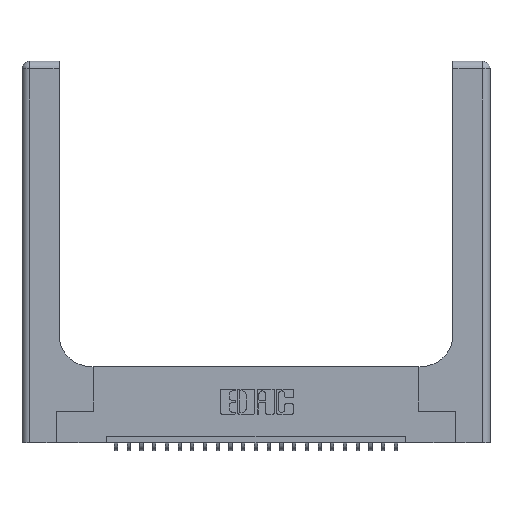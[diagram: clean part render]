
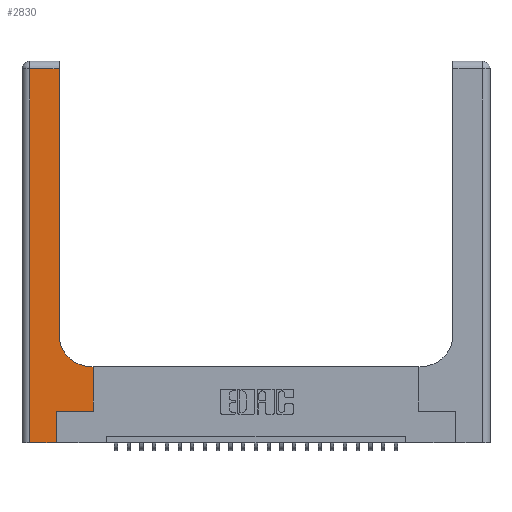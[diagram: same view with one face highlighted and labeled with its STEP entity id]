
A CAD part, top view. The second image highlights one B-rep face of the part: STEP entity #2830.
In plain terms, the highlighted planar face has unit normal (0, 0, 1).
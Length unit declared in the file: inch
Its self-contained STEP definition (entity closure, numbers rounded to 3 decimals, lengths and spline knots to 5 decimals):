
#222 = VERTEX_POINT ( 'NONE', #19089 ) ;
#286 = DIRECTION ( 'NONE',  ( 0., 1., 0. ) ) ;
#414 = CARTESIAN_POINT ( 'NONE',  ( 0.5415, 0.6, 0.37 ) ) ;
#593 = LINE ( 'NONE', #1407, #20966 ) ;
#1171 = CARTESIAN_POINT ( 'NONE',  ( 0.5585, 0.25, 0.37 ) ) ;
#1226 = FACE_OUTER_BOUND ( 'NONE', #12629, .T. ) ;
#1344 = LINE ( 'NONE', #21145, #14712 ) ;
#1407 = CARTESIAN_POINT ( 'NONE',  ( 0.06, 3., 0.37 ) ) ;
#2830 = ADVANCED_FACE ( 'NONE', ( #1226 ), #5696, .F. ) ;
#3647 = DIRECTION ( 'NONE',  ( -1., 0., 0. ) ) ;
#3951 = LINE ( 'NONE', #14547, #21245 ) ;
#5026 = ORIENTED_EDGE ( 'NONE', *, *, #21428, .T. ) ;
#5263 = VERTEX_POINT ( 'NONE', #8131 ) ;
#5564 = CARTESIAN_POINT ( 'NONE',  ( 0.5585, 0.25, 0.37 ) ) ;
#5696 = PLANE ( 'NONE',  #17674 ) ;
#5729 = ORIENTED_EDGE ( 'NONE', *, *, #15155, .T. ) ;
#6501 = VECTOR ( 'NONE', #286, 39.37008 ) ;
#6520 = LINE ( 'NONE', #1171, #6821 ) ;
#6821 = VECTOR ( 'NONE', #14760, 39.37008 ) ;
#7283 = EDGE_CURVE ( 'NONE', #222, #21308, #1344, .T. ) ;
#7438 = ORIENTED_EDGE ( 'NONE', *, *, #7283, .T. ) ;
#7565 = DIRECTION ( 'NONE',  ( 0., 0., -1. ) ) ;
#7624 = EDGE_CURVE ( 'NONE', #19038, #5263, #6520, .T. ) ;
#8131 = CARTESIAN_POINT ( 'NONE',  ( 0.5585, 0.6, 0.37 ) ) ;
#8692 = VERTEX_POINT ( 'NONE', #13277 ) ;
#9406 = CARTESIAN_POINT ( 'NONE',  ( 0., 0., 0.37 ) ) ;
#10143 = DIRECTION ( 'NONE',  ( 0., -1., 0. ) ) ;
#10182 = LINE ( 'NONE', #21748, #13171 ) ;
#10460 = ORIENTED_EDGE ( 'NONE', *, *, #20846, .T. ) ;
#11235 = DIRECTION ( 'NONE',  ( -1., 0., 0. ) ) ;
#12629 = EDGE_LOOP ( 'NONE', ( #7438, #10460, #18470, #15823, #5026, #5729, #13720, #17035, #15009 ) ) ;
#13171 = VECTOR ( 'NONE', #19708, 39.37008 ) ;
#13198 = LINE ( 'NONE', #13828, #19577 ) ;
#13277 = CARTESIAN_POINT ( 'NONE',  ( 0.06, 2.94, 0.37 ) ) ;
#13284 = CARTESIAN_POINT ( 'NONE',  ( 0., 3., 0.37 ) ) ;
#13365 = DIRECTION ( 'NONE',  ( 1., 0., 0. ) ) ;
#13601 = EDGE_CURVE ( 'NONE', #8692, #20129, #593, .T. ) ;
#13603 = CARTESIAN_POINT ( 'NONE',  ( 0.06, 0., 0.37 ) ) ;
#13720 = ORIENTED_EDGE ( 'NONE', *, *, #7624, .T. ) ;
#13828 = CARTESIAN_POINT ( 'NONE',  ( 0., 2.94, 0.37 ) ) ;
#14547 = CARTESIAN_POINT ( 'NONE',  ( 0.2915, 0.6, 0.37 ) ) ;
#14712 = VECTOR ( 'NONE', #22894, 39.37008 ) ;
#14760 = DIRECTION ( 'NONE',  ( 0., 1., 0. ) ) ;
#14888 = CARTESIAN_POINT ( 'NONE',  ( 0.269, 0., 0.37 ) ) ;
#15009 = ORIENTED_EDGE ( 'NONE', *, *, #15524, .T. ) ;
#15155 = EDGE_CURVE ( 'NONE', #17272, #19038, #10182, .T. ) ;
#15264 = VERTEX_POINT ( 'NONE', #414 ) ;
#15524 = EDGE_CURVE ( 'NONE', #15264, #222, #21955, .T. ) ;
#15766 = DIRECTION ( 'NONE',  ( -1., 0., 0. ) ) ;
#15823 = ORIENTED_EDGE ( 'NONE', *, *, #16827, .T. ) ;
#15845 = LINE ( 'NONE', #9406, #20418 ) ;
#16827 = EDGE_CURVE ( 'NONE', #20129, #23615, #15845, .T. ) ;
#17035 = ORIENTED_EDGE ( 'NONE', *, *, #18472, .T. ) ;
#17272 = VERTEX_POINT ( 'NONE', #20364 ) ;
#17674 = AXIS2_PLACEMENT_3D ( 'NONE', #13284, #7565, #3647 ) ;
#18016 = DIRECTION ( 'NONE',  ( 0., 0., -1. ) ) ;
#18470 = ORIENTED_EDGE ( 'NONE', *, *, #13601, .T. ) ;
#18472 = EDGE_CURVE ( 'NONE', #5263, #15264, #3951, .T. ) ;
#19038 = VERTEX_POINT ( 'NONE', #5564 ) ;
#19089 = CARTESIAN_POINT ( 'NONE',  ( 0.2915, 0.85, 0.37 ) ) ;
#19577 = VECTOR ( 'NONE', #15766, 39.37008 ) ;
#19708 = DIRECTION ( 'NONE',  ( 1., 0., 0. ) ) ;
#20124 = CARTESIAN_POINT ( 'NONE',  ( 0.5415, 0.85, 0.37 ) ) ;
#20129 = VERTEX_POINT ( 'NONE', #13603 ) ;
#20364 = CARTESIAN_POINT ( 'NONE',  ( 0.269, 0.25, 0.37 ) ) ;
#20418 = VECTOR ( 'NONE', #13365, 39.37008 ) ;
#20846 = EDGE_CURVE ( 'NONE', #21308, #8692, #13198, .T. ) ;
#20966 = VECTOR ( 'NONE', #10143, 39.37008 ) ;
#21145 = CARTESIAN_POINT ( 'NONE',  ( 0.2915, 3., 0.37 ) ) ;
#21245 = VECTOR ( 'NONE', #11235, 39.37008 ) ;
#21308 = VERTEX_POINT ( 'NONE', #21429 ) ;
#21428 = EDGE_CURVE ( 'NONE', #23615, #17272, #24983, .T. ) ;
#21429 = CARTESIAN_POINT ( 'NONE',  ( 0.2915, 2.94, 0.37 ) ) ;
#21500 = CARTESIAN_POINT ( 'NONE',  ( 0.269, 0., 0.37 ) ) ;
#21748 = CARTESIAN_POINT ( 'NONE',  ( 0.269, 0.25, 0.37 ) ) ;
#21955 = CIRCLE ( 'NONE', #23367, 0.25 ) ;
#22894 = DIRECTION ( 'NONE',  ( 0., 1., 0. ) ) ;
#23367 = AXIS2_PLACEMENT_3D ( 'NONE', #20124, #18016, #23856 ) ;
#23615 = VERTEX_POINT ( 'NONE', #14888 ) ;
#23856 = DIRECTION ( 'NONE',  ( 1., 0., 0. ) ) ;
#24983 = LINE ( 'NONE', #21500, #6501 ) ;
